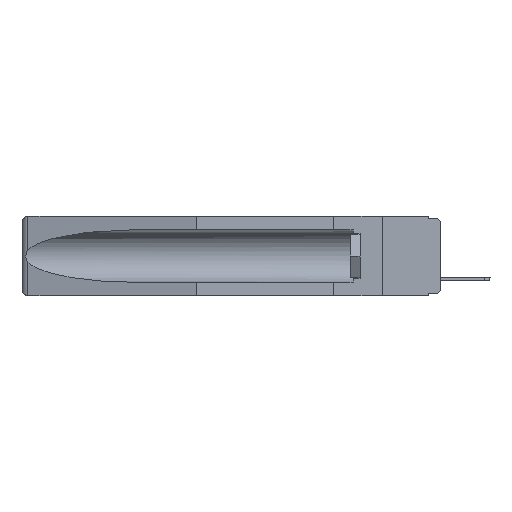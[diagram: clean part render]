
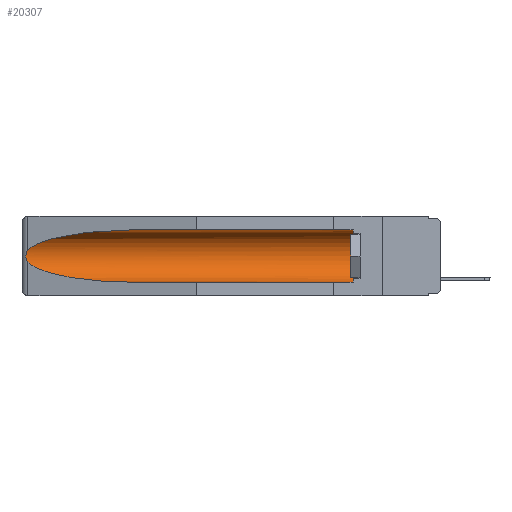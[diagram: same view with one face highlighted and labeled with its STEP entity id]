
A CAD part, left-side view. The second image highlights one B-rep face of the part: STEP entity #20307.
In plain terms, the highlighted cylindrical face has radius 2.857 mm (diameter 5.715 mm), a partial arc.
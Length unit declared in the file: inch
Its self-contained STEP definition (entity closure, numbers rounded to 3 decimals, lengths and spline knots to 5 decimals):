
#512 = CARTESIAN_POINT ( 'NONE',  ( 0.26654, 1.53092, -0.15636 ) ) ;
#822 = CARTESIAN_POINT ( 'NONE',  ( 0.21114, 1.30732, -0.059 ) ) ;
#967 =( BOUNDED_CURVE ( )  B_SPLINE_CURVE ( 3, ( #5590, #12661, #17738, #12779 ),
 .UNSPECIFIED., .F., .T. ) 
 B_SPLINE_CURVE_WITH_KNOTS ( ( 4, 4 ),
 ( 0.1948, 1.5708 ),
 .UNSPECIFIED. ) 
 CURVE ( )  GEOMETRIC_REPRESENTATION_ITEM ( )  RATIONAL_B_SPLINE_CURVE ( ( 1., 0.848, 0.848, 1. ) ) 
 REPRESENTATION_ITEM ( '' )  );
#1001 = DIRECTION ( 'NONE',  ( 0., 0., 1. ) ) ;
#1015 = CARTESIAN_POINT ( 'NONE',  ( 0.155, -0.30754, -0.284 ) ) ;
#2093 = AXIS2_PLACEMENT_3D ( 'NONE', #6172, #13156, #1001 ) ;
#2191 = FACE_OUTER_BOUND ( 'NONE', #18448, .T. ) ;
#2194 = VERTEX_POINT ( 'NONE', #5885 ) ;
#2315 = CARTESIAN_POINT ( 'NONE',  ( 0.155, -0.30754, -0.059 ) ) ;
#2664 = VERTEX_POINT ( 'NONE', #21403 ) ;
#3886 = B_SPLINE_CURVE_WITH_KNOTS ( 'NONE', 3,
 ( #20891, #21009, #512, #10635, #15927, #12544, #21123, #3994, #17504, #7154 ),
 .UNSPECIFIED., .F., .F.,
 ( 4, 2, 2, 2, 4 ),
 ( 0., 0.00029, 0.00058, 0.00087, 0.00117 ),
 .UNSPECIFIED. ) ;
#3926 = VECTOR ( 'NONE', #5261, 39.37008 ) ;
#3994 = CARTESIAN_POINT ( 'NONE',  ( 0.26655, 1.53094, -0.18657 ) ) ;
#4717 = VERTEX_POINT ( 'NONE', #12825 ) ;
#4748 = CARTESIAN_POINT ( 'NONE',  ( 0.26537, 1.52718, -0.14972 ) ) ;
#5261 = DIRECTION ( 'NONE',  ( 0., 1., 0. ) ) ;
#5336 = CIRCLE ( 'NONE', #2093, 0.1125 ) ;
#5362 = CARTESIAN_POINT ( 'NONE',  ( 0.155, 0.126, -0.059 ) ) ;
#5474 = EDGE_CURVE ( 'NONE', #2664, #4717, #3886, .T. ) ;
#5479 = VERTEX_POINT ( 'NONE', #13907 ) ;
#5590 = CARTESIAN_POINT ( 'NONE',  ( 0.26537, 1.52718, -0.19328 ) ) ;
#5885 = CARTESIAN_POINT ( 'NONE',  ( 0.155, 1.07973, -0.284 ) ) ;
#6172 = CARTESIAN_POINT ( 'NONE',  ( 0.155, 0.126, -0.1715 ) ) ;
#6908 = VECTOR ( 'NONE', #10235, 39.37008 ) ;
#7154 = CARTESIAN_POINT ( 'NONE',  ( 0.26537, 1.52718, -0.19328 ) ) ;
#9274 = DIRECTION ( 'NONE',  ( 0., 1., 0. ) ) ;
#9861 = ORIENTED_EDGE ( 'NONE', *, *, #18838, .F. ) ;
#10235 = DIRECTION ( 'NONE',  ( 0., 1., 0. ) ) ;
#10524 = AXIS2_PLACEMENT_3D ( 'NONE', #17511, #9274, #10643 ) ;
#10635 = CARTESIAN_POINT ( 'NONE',  ( 0.2673, 1.5327, -0.16383 ) ) ;
#10643 = DIRECTION ( 'NONE',  ( 0., 0., 1. ) ) ;
#11343 = VERTEX_POINT ( 'NONE', #22146 ) ;
#11398 = CARTESIAN_POINT ( 'NONE',  ( 0.155, 1.07973, -0.059 ) ) ;
#11783 =( BOUNDED_CURVE ( )  B_SPLINE_CURVE ( 3, ( #11398, #822, #14770, #4748 ),
 .UNSPECIFIED., .F., .T. ) 
 B_SPLINE_CURVE_WITH_KNOTS ( ( 4, 4 ),
 ( 4.71239, 6.08839 ),
 .UNSPECIFIED. ) 
 CURVE ( )  GEOMETRIC_REPRESENTATION_ITEM ( )  RATIONAL_B_SPLINE_CURVE ( ( 1., 0.848, 0.848, 1. ) ) 
 REPRESENTATION_ITEM ( '' )  );
#12327 = CYLINDRICAL_SURFACE ( 'NONE', #10524, 0.1125 ) ;
#12544 = CARTESIAN_POINT ( 'NONE',  ( 0.2675, 1.53308, -0.17534 ) ) ;
#12661 = CARTESIAN_POINT ( 'NONE',  ( 0.25451, 1.48313, -0.24835 ) ) ;
#12779 = CARTESIAN_POINT ( 'NONE',  ( 0.155, 1.07973, -0.284 ) ) ;
#12825 = CARTESIAN_POINT ( 'NONE',  ( 0.26537, 1.52718, -0.19328 ) ) ;
#12981 = EDGE_CURVE ( 'NONE', #20205, #11343, #14029, .T. ) ;
#13156 = DIRECTION ( 'NONE',  ( 0., -1., 0. ) ) ;
#13907 = CARTESIAN_POINT ( 'NONE',  ( 0.155, 0.126, -0.284 ) ) ;
#13950 = ORIENTED_EDGE ( 'NONE', *, *, #22175, .T. ) ;
#13958 = EDGE_CURVE ( 'NONE', #5479, #20205, #5336, .T. ) ;
#14029 = LINE ( 'NONE', #2315, #3926 ) ;
#14633 = ORIENTED_EDGE ( 'NONE', *, *, #5474, .T. ) ;
#14770 = CARTESIAN_POINT ( 'NONE',  ( 0.25451, 1.48313, -0.09465 ) ) ;
#15927 = CARTESIAN_POINT ( 'NONE',  ( 0.2675, 1.53308, -0.16763 ) ) ;
#16443 = LINE ( 'NONE', #1015, #6908 ) ;
#16911 = ORIENTED_EDGE ( 'NONE', *, *, #13958, .T. ) ;
#17504 = CARTESIAN_POINT ( 'NONE',  ( 0.26597, 1.5296, -0.19026 ) ) ;
#17511 = CARTESIAN_POINT ( 'NONE',  ( 0.155, -0.30754, -0.1715 ) ) ;
#17738 = CARTESIAN_POINT ( 'NONE',  ( 0.21114, 1.30732, -0.284 ) ) ;
#18168 = ORIENTED_EDGE ( 'NONE', *, *, #20216, .T. ) ;
#18448 = EDGE_LOOP ( 'NONE', ( #13950, #14633, #18168, #9861, #16911, #21976 ) ) ;
#18838 = EDGE_CURVE ( 'NONE', #5479, #2194, #16443, .T. ) ;
#20205 = VERTEX_POINT ( 'NONE', #5362 ) ;
#20216 = EDGE_CURVE ( 'NONE', #4717, #2194, #967, .T. ) ;
#20307 = ADVANCED_FACE ( 'NONE', ( #2191 ), #12327, .F. ) ;
#20891 = CARTESIAN_POINT ( 'NONE',  ( 0.26537, 1.52718, -0.14972 ) ) ;
#21009 = CARTESIAN_POINT ( 'NONE',  ( 0.26597, 1.52961, -0.15275 ) ) ;
#21123 = CARTESIAN_POINT ( 'NONE',  ( 0.2673, 1.53269, -0.17917 ) ) ;
#21403 = CARTESIAN_POINT ( 'NONE',  ( 0.26537, 1.52718, -0.14972 ) ) ;
#21976 = ORIENTED_EDGE ( 'NONE', *, *, #12981, .T. ) ;
#22146 = CARTESIAN_POINT ( 'NONE',  ( 0.155, 1.07973, -0.059 ) ) ;
#22175 = EDGE_CURVE ( 'NONE', #11343, #2664, #11783, .T. ) ;
